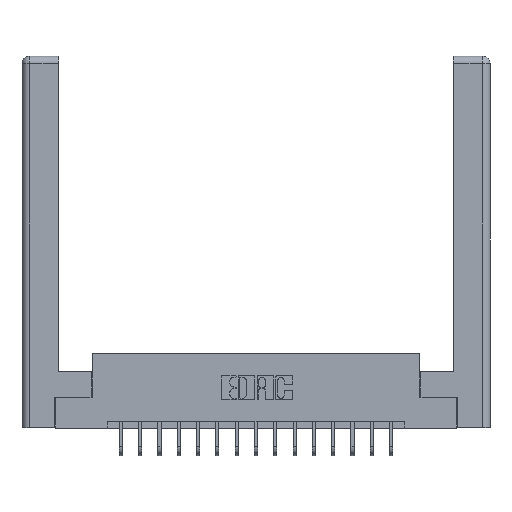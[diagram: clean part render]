
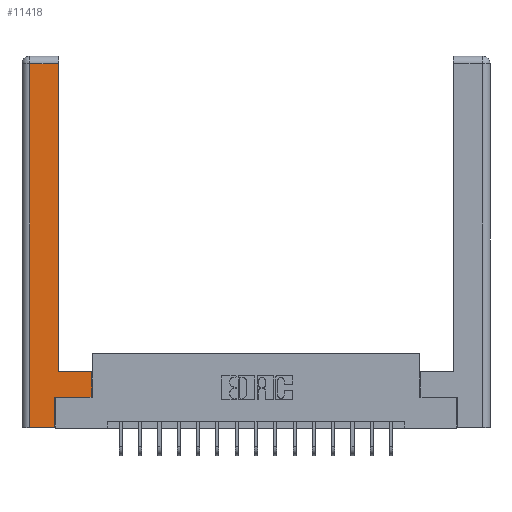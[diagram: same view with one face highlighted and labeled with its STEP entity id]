
A CAD part, top view. The second image highlights one B-rep face of the part: STEP entity #11418.
In plain terms, the highlighted planar face has unit normal (0, 0, 1).
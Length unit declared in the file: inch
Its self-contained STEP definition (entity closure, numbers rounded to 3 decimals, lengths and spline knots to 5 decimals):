
#242 = ORIENTED_EDGE ( 'NONE', *, *, #19246, .T. ) ;
#797 = DIRECTION ( 'NONE',  ( 0., 1., 0. ) ) ;
#1664 = ORIENTED_EDGE ( 'NONE', *, *, #8332, .T. ) ;
#1857 = VERTEX_POINT ( 'NONE', #14802 ) ;
#2248 = VECTOR ( 'NONE', #17521, 39.37008 ) ;
#2446 = VECTOR ( 'NONE', #797, 39.37008 ) ;
#2527 = CARTESIAN_POINT ( 'NONE',  ( 0.295, 3., 0. ) ) ;
#2795 = ORIENTED_EDGE ( 'NONE', *, *, #12025, .T. ) ;
#3479 = VECTOR ( 'NONE', #6762, 39.37008 ) ;
#3547 = CARTESIAN_POINT ( 'NONE',  ( 0.265, 0.245, 0. ) ) ;
#3763 = CARTESIAN_POINT ( 'NONE',  ( 0.295, 2.94, 0. ) ) ;
#3833 = CARTESIAN_POINT ( 'NONE',  ( 0., 0., 0. ) ) ;
#3895 = LINE ( 'NONE', #2527, #2446 ) ;
#3943 = CARTESIAN_POINT ( 'NONE',  ( 0.0615, 0., 0. ) ) ;
#3973 = LINE ( 'NONE', #14064, #17398 ) ;
#4069 = DIRECTION ( 'NONE',  ( 1., 0., 0. ) ) ;
#4163 = CARTESIAN_POINT ( 'NONE',  ( 0.565, 0.45, 0. ) ) ;
#4206 = CARTESIAN_POINT ( 'NONE',  ( 0.565, 0.245, 0. ) ) ;
#4355 = CARTESIAN_POINT ( 'NONE',  ( 0.0615, 0., 0. ) ) ;
#5009 = EDGE_CURVE ( 'NONE', #10628, #17571, #18099, .T. ) ;
#6094 = DIRECTION ( 'NONE',  ( 1., 0., 0. ) ) ;
#6364 = EDGE_CURVE ( 'NONE', #16654, #1857, #19244, .T. ) ;
#6697 = VECTOR ( 'NONE', #19506, 39.37008 ) ;
#6750 = ORIENTED_EDGE ( 'NONE', *, *, #6364, .T. ) ;
#6762 = DIRECTION ( 'NONE',  ( 0., 1., 0. ) ) ;
#6875 = EDGE_LOOP ( 'NONE', ( #17236, #2795, #14122, #15825, #9506, #1664, #6750, #242 ) ) ;
#6908 = EDGE_CURVE ( 'NONE', #15202, #14910, #3895, .T. ) ;
#7382 = CARTESIAN_POINT ( 'NONE',  ( 0.295, 0.45, 0. ) ) ;
#8129 = CARTESIAN_POINT ( 'NONE',  ( 0.265, 0.245, 0. ) ) ;
#8165 = AXIS2_PLACEMENT_3D ( 'NONE', #3833, #19053, #13318 ) ;
#8247 = VERTEX_POINT ( 'NONE', #3943 ) ;
#8332 = EDGE_CURVE ( 'NONE', #17571, #16654, #8536, .T. ) ;
#8536 = LINE ( 'NONE', #4206, #17030 ) ;
#8812 = CARTESIAN_POINT ( 'NONE',  ( 0.295, 0.45, 0. ) ) ;
#8930 = CARTESIAN_POINT ( 'NONE',  ( 0.0615, 2.94, 0. ) ) ;
#9506 = ORIENTED_EDGE ( 'NONE', *, *, #5009, .T. ) ;
#10072 = EDGE_CURVE ( 'NONE', #8247, #10628, #14185, .T. ) ;
#10628 = VERTEX_POINT ( 'NONE', #17363 ) ;
#11418 = ADVANCED_FACE ( 'NONE', ( #14843 ), #12863, .F. ) ;
#12025 = EDGE_CURVE ( 'NONE', #14910, #14279, #3973, .T. ) ;
#12863 = PLANE ( 'NONE',  #8165 ) ;
#13252 = VECTOR ( 'NONE', #6094, 39.37008 ) ;
#13318 = DIRECTION ( 'NONE',  ( -1., 0., 0. ) ) ;
#13864 = CARTESIAN_POINT ( 'NONE',  ( 0.565, 0.245, 0. ) ) ;
#14064 = CARTESIAN_POINT ( 'NONE',  ( 0.0615, 2.94, 0. ) ) ;
#14122 = ORIENTED_EDGE ( 'NONE', *, *, #15149, .T. ) ;
#14185 = LINE ( 'NONE', #18066, #13252 ) ;
#14279 = VERTEX_POINT ( 'NONE', #8930 ) ;
#14802 = CARTESIAN_POINT ( 'NONE',  ( 0.565, 0.45, 0. ) ) ;
#14843 = FACE_OUTER_BOUND ( 'NONE', #6875, .T. ) ;
#14910 = VERTEX_POINT ( 'NONE', #3763 ) ;
#15149 = EDGE_CURVE ( 'NONE', #14279, #8247, #16561, .T. ) ;
#15202 = VERTEX_POINT ( 'NONE', #8812 ) ;
#15582 = DIRECTION ( 'NONE',  ( -1., 0., 0. ) ) ;
#15825 = ORIENTED_EDGE ( 'NONE', *, *, #10072, .T. ) ;
#16074 = VECTOR ( 'NONE', #19308, 39.37008 ) ;
#16561 = LINE ( 'NONE', #4355, #16074 ) ;
#16654 = VERTEX_POINT ( 'NONE', #13864 ) ;
#17030 = VECTOR ( 'NONE', #4069, 39.37008 ) ;
#17236 = ORIENTED_EDGE ( 'NONE', *, *, #6908, .T. ) ;
#17363 = CARTESIAN_POINT ( 'NONE',  ( 0.265, 0., 0. ) ) ;
#17398 = VECTOR ( 'NONE', #15582, 39.37008 ) ;
#17521 = DIRECTION ( 'NONE',  ( 0., 1., 0. ) ) ;
#17571 = VERTEX_POINT ( 'NONE', #3547 ) ;
#18066 = CARTESIAN_POINT ( 'NONE',  ( 0.265, 0., 0. ) ) ;
#18099 = LINE ( 'NONE', #8129, #3479 ) ;
#19053 = DIRECTION ( 'NONE',  ( 0., 0., -1. ) ) ;
#19181 = LINE ( 'NONE', #7382, #6697 ) ;
#19244 = LINE ( 'NONE', #4163, #2248 ) ;
#19246 = EDGE_CURVE ( 'NONE', #1857, #15202, #19181, .T. ) ;
#19308 = DIRECTION ( 'NONE',  ( 0., -1., 0. ) ) ;
#19506 = DIRECTION ( 'NONE',  ( -1., 0., 0. ) ) ;
